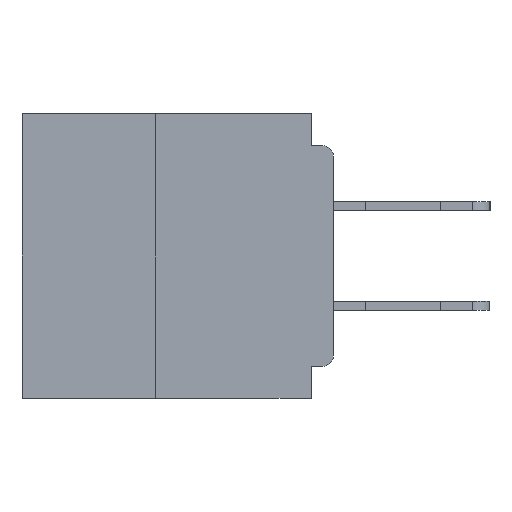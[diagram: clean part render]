
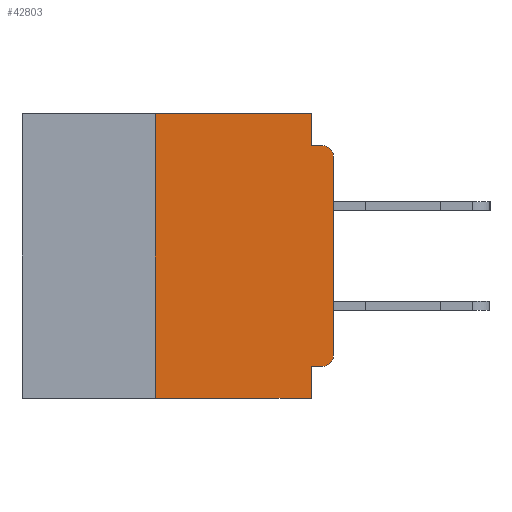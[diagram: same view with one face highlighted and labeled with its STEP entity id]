
A CAD part, left-side view. The second image highlights one B-rep face of the part: STEP entity #42803.
In plain terms, the highlighted planar face has unit normal (-1, 0, 0).
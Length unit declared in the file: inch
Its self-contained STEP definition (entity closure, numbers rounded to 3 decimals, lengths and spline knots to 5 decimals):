
#554 = CARTESIAN_POINT ( 'NONE',  ( 0., 0.031, -0.045 ) ) ;
#636 = PLANE ( 'NONE',  #40775 ) ;
#801 = LINE ( 'NONE', #26205, #9218 ) ;
#1089 = LINE ( 'NONE', #6740, #28087 ) ;
#1258 = VERTEX_POINT ( 'NONE', #12763 ) ;
#1390 = VERTEX_POINT ( 'NONE', #22910 ) ;
#1835 = CARTESIAN_POINT ( 'NONE',  ( 0., 0.031, -0.4 ) ) ;
#2418 = CARTESIAN_POINT ( 'NONE',  ( 0., 0.031, -0.355 ) ) ;
#3096 = EDGE_CURVE ( 'NONE', #21502, #1258, #40914, .T. ) ;
#3344 = AXIS2_PLACEMENT_3D ( 'NONE', #9018, #33561, #12593 ) ;
#3836 = ORIENTED_EDGE ( 'NONE', *, *, #3096, .T. ) ;
#4656 = CARTESIAN_POINT ( 'NONE',  ( 0., 0.437, -0.4 ) ) ;
#4939 = DIRECTION ( 'NONE',  ( -1., 0., 0. ) ) ;
#6412 = LINE ( 'NONE', #31459, #22916 ) ;
#6740 = CARTESIAN_POINT ( 'NONE',  ( 0., 0.25, -0.4 ) ) ;
#6745 = CARTESIAN_POINT ( 'NONE',  ( 0., 0.031, 0. ) ) ;
#6854 = LINE ( 'NONE', #19351, #16294 ) ;
#9018 = CARTESIAN_POINT ( 'NONE',  ( 0., 0.015, -0.06 ) ) ;
#9218 = VECTOR ( 'NONE', #36829, 39.37008 ) ;
#10081 = AXIS2_PLACEMENT_3D ( 'NONE', #26006, #4939, #29536 ) ;
#10365 = DIRECTION ( 'NONE',  ( 0., 0., -1. ) ) ;
#11561 = DIRECTION ( 'NONE',  ( 1., 0., 0. ) ) ;
#11796 = CARTESIAN_POINT ( 'NONE',  ( 0., 0.25, 0. ) ) ;
#12593 = DIRECTION ( 'NONE',  ( 0., 0., -1. ) ) ;
#12763 = CARTESIAN_POINT ( 'NONE',  ( 0., 0.015, -0.045 ) ) ;
#13134 = VERTEX_POINT ( 'NONE', #1835 ) ;
#14411 = LINE ( 'NONE', #16987, #31898 ) ;
#15696 = VERTEX_POINT ( 'NONE', #554 ) ;
#15839 = ORIENTED_EDGE ( 'NONE', *, *, #38231, .F. ) ;
#16020 = CARTESIAN_POINT ( 'NONE',  ( 0., 0.015, -0.355 ) ) ;
#16294 = VECTOR ( 'NONE', #33456, 39.37008 ) ;
#16579 = EDGE_CURVE ( 'NONE', #44427, #21502, #801, .T. ) ;
#16987 = CARTESIAN_POINT ( 'NONE',  ( 0., 0.031, -0.4 ) ) ;
#17038 = EDGE_CURVE ( 'NONE', #35371, #15696, #45307, .T. ) ;
#17672 = CARTESIAN_POINT ( 'NONE',  ( 0., 0.437, 0. ) ) ;
#17907 = EDGE_CURVE ( 'NONE', #1390, #13134, #33777, .T. ) ;
#19169 = ORIENTED_EDGE ( 'NONE', *, *, #17038, .F. ) ;
#19351 = CARTESIAN_POINT ( 'NONE',  ( 0., 0., -0.355 ) ) ;
#20474 = DIRECTION ( 'NONE',  ( 0., 0., -1. ) ) ;
#21151 = DIRECTION ( 'NONE',  ( 0., -1., 0. ) ) ;
#21345 = EDGE_LOOP ( 'NONE', ( #43873, #3836, #32158, #19169, #36775, #27003, #41797, #36079, #15839, #33417 ) ) ;
#21502 = VERTEX_POINT ( 'NONE', #29819 ) ;
#22900 = EDGE_CURVE ( 'NONE', #27618, #44427, #41490, .T. ) ;
#22910 = CARTESIAN_POINT ( 'NONE',  ( 0., 0.25, -0.4 ) ) ;
#22916 = VECTOR ( 'NONE', #34996, 39.37008 ) ;
#24391 = VECTOR ( 'NONE', #25877, 39.37008 ) ;
#25877 = DIRECTION ( 'NONE',  ( 0., -1., 0. ) ) ;
#26006 = CARTESIAN_POINT ( 'NONE',  ( 0., 0.015, -0.34 ) ) ;
#26205 = CARTESIAN_POINT ( 'NONE',  ( 0., 0., 0. ) ) ;
#26825 = VERTEX_POINT ( 'NONE', #11796 ) ;
#27003 = ORIENTED_EDGE ( 'NONE', *, *, #27241, .F. ) ;
#27241 = EDGE_CURVE ( 'NONE', #1390, #26825, #1089, .T. ) ;
#27618 = VERTEX_POINT ( 'NONE', #16020 ) ;
#28087 = VECTOR ( 'NONE', #41873, 39.37008 ) ;
#29536 = DIRECTION ( 'NONE',  ( 0., 0., -1. ) ) ;
#29819 = CARTESIAN_POINT ( 'NONE',  ( 0., 0., -0.06 ) ) ;
#30697 = CARTESIAN_POINT ( 'NONE',  ( 0., 0., -0.34 ) ) ;
#30975 = LINE ( 'NONE', #17672, #39201 ) ;
#31459 = CARTESIAN_POINT ( 'NONE',  ( 0., 0., -0.045 ) ) ;
#31898 = VECTOR ( 'NONE', #20474, 39.37008 ) ;
#32158 = ORIENTED_EDGE ( 'NONE', *, *, #42610, .F. ) ;
#32533 = CARTESIAN_POINT ( 'NONE',  ( 0., 0.437, 0. ) ) ;
#33417 = ORIENTED_EDGE ( 'NONE', *, *, #22900, .T. ) ;
#33456 = DIRECTION ( 'NONE',  ( 0., 1., 0. ) ) ;
#33487 = EDGE_CURVE ( 'NONE', #26825, #35371, #30975, .T. ) ;
#33561 = DIRECTION ( 'NONE',  ( -1., 0., 0. ) ) ;
#33777 = LINE ( 'NONE', #4656, #24391 ) ;
#34936 = VECTOR ( 'NONE', #10365, 39.37008 ) ;
#34996 = DIRECTION ( 'NONE',  ( 0., -1., 0. ) ) ;
#35206 = EDGE_CURVE ( 'NONE', #39023, #13134, #14411, .T. ) ;
#35371 = VERTEX_POINT ( 'NONE', #35488 ) ;
#35488 = CARTESIAN_POINT ( 'NONE',  ( 0., 0.031, 0. ) ) ;
#36066 = DIRECTION ( 'NONE',  ( 0., 0., -1. ) ) ;
#36079 = ORIENTED_EDGE ( 'NONE', *, *, #35206, .F. ) ;
#36775 = ORIENTED_EDGE ( 'NONE', *, *, #33487, .F. ) ;
#36829 = DIRECTION ( 'NONE',  ( 0., 0., 1. ) ) ;
#38231 = EDGE_CURVE ( 'NONE', #27618, #39023, #6854, .T. ) ;
#39023 = VERTEX_POINT ( 'NONE', #2418 ) ;
#39201 = VECTOR ( 'NONE', #21151, 39.37008 ) ;
#40775 = AXIS2_PLACEMENT_3D ( 'NONE', #32533, #11561, #36066 ) ;
#40914 = CIRCLE ( 'NONE', #3344, 0.015 ) ;
#40993 = FACE_OUTER_BOUND ( 'NONE', #21345, .T. ) ;
#41490 = CIRCLE ( 'NONE', #10081, 0.015 ) ;
#41797 = ORIENTED_EDGE ( 'NONE', *, *, #17907, .T. ) ;
#41873 = DIRECTION ( 'NONE',  ( 0., 0., 1. ) ) ;
#42610 = EDGE_CURVE ( 'NONE', #15696, #1258, #6412, .T. ) ;
#42803 = ADVANCED_FACE ( 'NONE', ( #40993 ), #636, .F. ) ;
#43873 = ORIENTED_EDGE ( 'NONE', *, *, #16579, .T. ) ;
#44427 = VERTEX_POINT ( 'NONE', #30697 ) ;
#45307 = LINE ( 'NONE', #6745, #34936 ) ;
